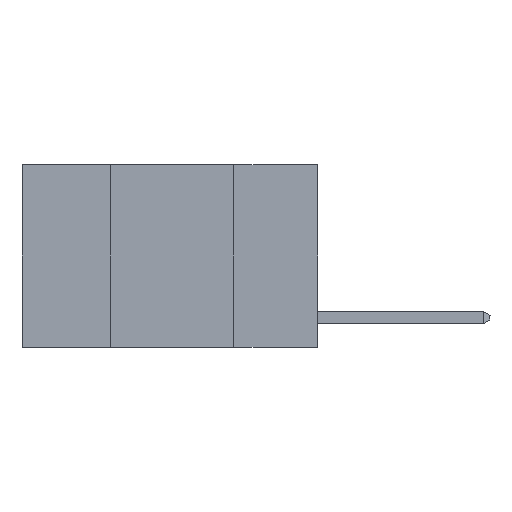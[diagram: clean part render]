
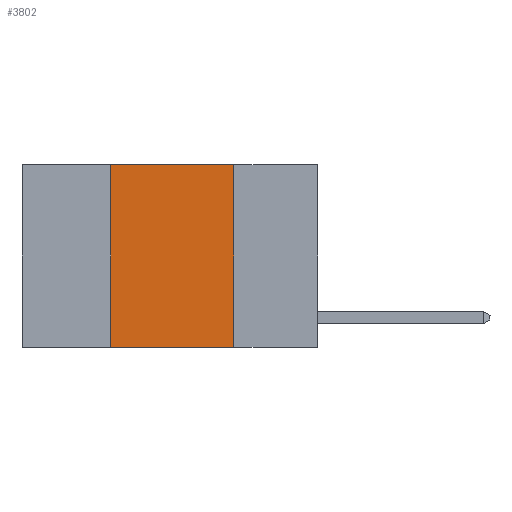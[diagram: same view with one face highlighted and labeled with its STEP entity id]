
A CAD part, left-side view. The second image highlights one B-rep face of the part: STEP entity #3802.
In plain terms, the highlighted planar face has unit normal (-1, 0, 0).
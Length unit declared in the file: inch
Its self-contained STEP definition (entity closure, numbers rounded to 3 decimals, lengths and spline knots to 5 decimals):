
#268 = CARTESIAN_POINT ( 'NONE',  ( 0., 0.17, -0.37 ) ) ;
#1184 = FACE_OUTER_BOUND ( 'NONE', #3898, .T. ) ;
#1565 = EDGE_CURVE ( 'NONE', #8076, #16163, #16914, .T. ) ;
#1684 = AXIS2_PLACEMENT_3D ( 'NONE', #16280, #13777, #7977 ) ;
#2703 = PLANE ( 'NONE',  #1684 ) ;
#3612 = EDGE_CURVE ( 'NONE', #9052, #17030, #11396, .T. ) ;
#3635 = CARTESIAN_POINT ( 'NONE',  ( 0., 0.17, 0. ) ) ;
#3802 = ADVANCED_FACE ( 'NONE', ( #1184 ), #2703, .F. ) ;
#3898 = EDGE_LOOP ( 'NONE', ( #4000, #14430, #10340, #6106 ) ) ;
#4000 = ORIENTED_EDGE ( 'NONE', *, *, #13937, .F. ) ;
#4185 = CARTESIAN_POINT ( 'NONE',  ( 0., 0.17, 0. ) ) ;
#5258 = EDGE_CURVE ( 'NONE', #9052, #8076, #6263, .T. ) ;
#5645 = CARTESIAN_POINT ( 'NONE',  ( 0., 0.42, 0. ) ) ;
#5940 = VECTOR ( 'NONE', #6355, 39.37008 ) ;
#6106 = ORIENTED_EDGE ( 'NONE', *, *, #3612, .T. ) ;
#6263 = LINE ( 'NONE', #10174, #5940 ) ;
#6272 = CARTESIAN_POINT ( 'NONE',  ( 0., 0.6, 0. ) ) ;
#6355 = DIRECTION ( 'NONE',  ( 0., 0., 1. ) ) ;
#7350 = VECTOR ( 'NONE', #7381, 39.37008 ) ;
#7381 = DIRECTION ( 'NONE',  ( 0., -1., 0. ) ) ;
#7977 = DIRECTION ( 'NONE',  ( 0., 0., -1. ) ) ;
#8076 = VERTEX_POINT ( 'NONE', #5645 ) ;
#8424 = VECTOR ( 'NONE', #14412, 39.37008 ) ;
#8591 = VECTOR ( 'NONE', #10270, 39.37008 ) ;
#9052 = VERTEX_POINT ( 'NONE', #15192 ) ;
#10174 = CARTESIAN_POINT ( 'NONE',  ( 0., 0.42, 0. ) ) ;
#10224 = LINE ( 'NONE', #3635, #8424 ) ;
#10270 = DIRECTION ( 'NONE',  ( 0., -1., 0. ) ) ;
#10340 = ORIENTED_EDGE ( 'NONE', *, *, #5258, .F. ) ;
#11396 = LINE ( 'NONE', #17245, #7350 ) ;
#13777 = DIRECTION ( 'NONE',  ( 1., 0., 0. ) ) ;
#13937 = EDGE_CURVE ( 'NONE', #16163, #17030, #10224, .T. ) ;
#14412 = DIRECTION ( 'NONE',  ( 0., 0., -1. ) ) ;
#14430 = ORIENTED_EDGE ( 'NONE', *, *, #1565, .F. ) ;
#15192 = CARTESIAN_POINT ( 'NONE',  ( 0., 0.42, -0.37 ) ) ;
#16163 = VERTEX_POINT ( 'NONE', #4185 ) ;
#16280 = CARTESIAN_POINT ( 'NONE',  ( 0., 0.6, 0. ) ) ;
#16914 = LINE ( 'NONE', #6272, #8591 ) ;
#17030 = VERTEX_POINT ( 'NONE', #268 ) ;
#17245 = CARTESIAN_POINT ( 'NONE',  ( 0., 0.6, -0.37 ) ) ;
